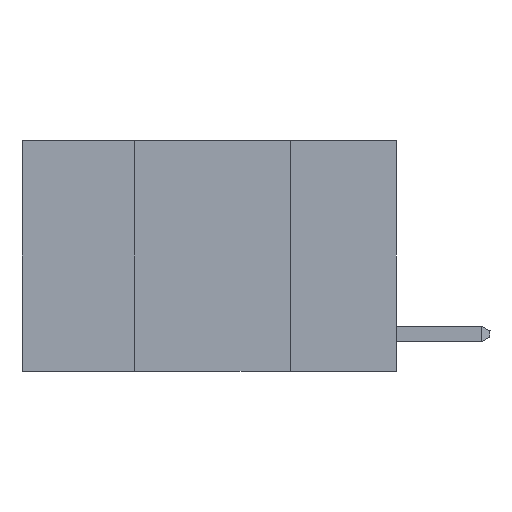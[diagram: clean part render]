
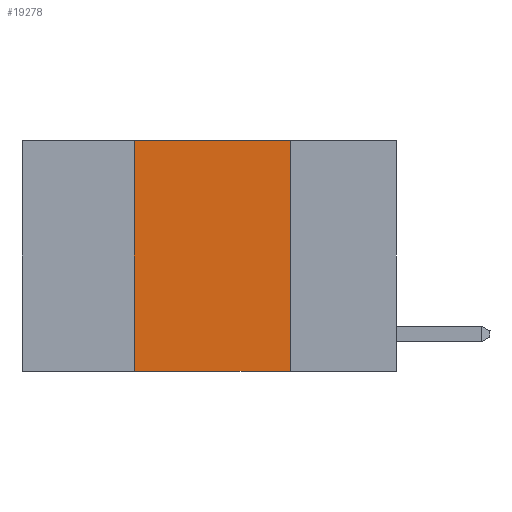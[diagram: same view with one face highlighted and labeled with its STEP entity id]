
A CAD part, left-side view. The second image highlights one B-rep face of the part: STEP entity #19278.
In plain terms, the highlighted planar face has unit normal (-1, 0, 0).
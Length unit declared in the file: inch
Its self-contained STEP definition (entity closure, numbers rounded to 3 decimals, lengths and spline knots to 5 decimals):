
#4096 = CARTESIAN_POINT ( 'NONE',  ( 0., 0.6, 0. ) ) ;
#4221 = DIRECTION ( 'NONE',  ( 0., 0., 1. ) ) ;
#5902 = VECTOR ( 'NONE', #4221, 39.37008 ) ;
#6093 = DIRECTION ( 'NONE',  ( 0., 0., -1. ) ) ;
#6629 = EDGE_CURVE ( 'NONE', #19640, #17079, #20900, .T. ) ;
#6995 = EDGE_CURVE ( 'NONE', #19640, #9180, #13017, .T. ) ;
#8852 = DIRECTION ( 'NONE',  ( 1., 0., 0. ) ) ;
#9180 = VERTEX_POINT ( 'NONE', #21869 ) ;
#10468 = ORIENTED_EDGE ( 'NONE', *, *, #25017, .F. ) ;
#11163 = FACE_OUTER_BOUND ( 'NONE', #23225, .T. ) ;
#11291 = DIRECTION ( 'NONE',  ( 0., -1., 0. ) ) ;
#13017 = LINE ( 'NONE', #18079, #29015 ) ;
#15817 = VECTOR ( 'NONE', #22033, 39.37008 ) ;
#15861 = LINE ( 'NONE', #4096, #18465 ) ;
#17079 = VERTEX_POINT ( 'NONE', #23501 ) ;
#17275 = VERTEX_POINT ( 'NONE', #23828 ) ;
#17963 = ORIENTED_EDGE ( 'NONE', *, *, #18739, .F. ) ;
#18079 = CARTESIAN_POINT ( 'NONE',  ( 0., 0.6, -0.37 ) ) ;
#18465 = VECTOR ( 'NONE', #27413, 39.37008 ) ;
#18739 = EDGE_CURVE ( 'NONE', #17079, #17275, #15861, .T. ) ;
#19278 = ADVANCED_FACE ( 'NONE', ( #11163 ), #30005, .F. ) ;
#19640 = VERTEX_POINT ( 'NONE', #24731 ) ;
#19955 = AXIS2_PLACEMENT_3D ( 'NONE', #27702, #8852, #6093 ) ;
#20588 = CARTESIAN_POINT ( 'NONE',  ( 0., 0.42, 0. ) ) ;
#20900 = LINE ( 'NONE', #20588, #5902 ) ;
#21869 = CARTESIAN_POINT ( 'NONE',  ( 0., 0.17, -0.37 ) ) ;
#22033 = DIRECTION ( 'NONE',  ( 0., 0., -1. ) ) ;
#23225 = EDGE_LOOP ( 'NONE', ( #10468, #17963, #30239, #27227 ) ) ;
#23501 = CARTESIAN_POINT ( 'NONE',  ( 0., 0.42, 0. ) ) ;
#23828 = CARTESIAN_POINT ( 'NONE',  ( 0., 0.17, 0. ) ) ;
#24224 = CARTESIAN_POINT ( 'NONE',  ( 0., 0.17, 0. ) ) ;
#24374 = LINE ( 'NONE', #24224, #15817 ) ;
#24731 = CARTESIAN_POINT ( 'NONE',  ( 0., 0.42, -0.37 ) ) ;
#25017 = EDGE_CURVE ( 'NONE', #17275, #9180, #24374, .T. ) ;
#27227 = ORIENTED_EDGE ( 'NONE', *, *, #6995, .T. ) ;
#27413 = DIRECTION ( 'NONE',  ( 0., -1., 0. ) ) ;
#27702 = CARTESIAN_POINT ( 'NONE',  ( 0., 0.6, 0. ) ) ;
#29015 = VECTOR ( 'NONE', #11291, 39.37008 ) ;
#30005 = PLANE ( 'NONE',  #19955 ) ;
#30239 = ORIENTED_EDGE ( 'NONE', *, *, #6629, .F. ) ;
